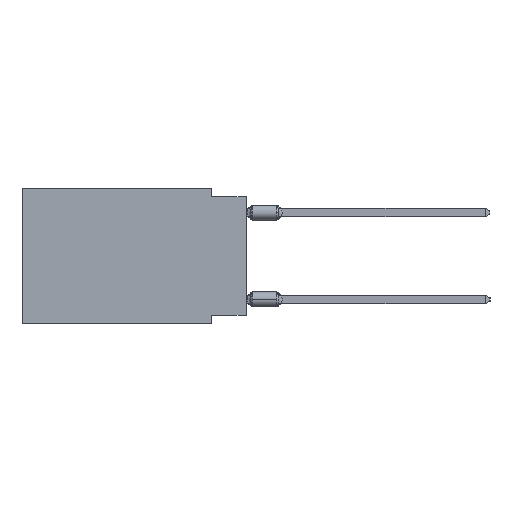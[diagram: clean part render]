
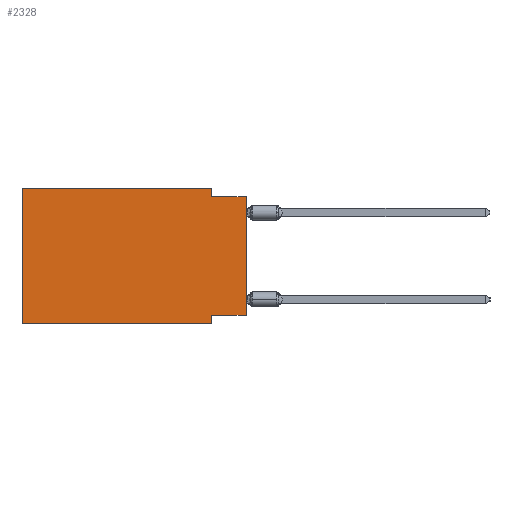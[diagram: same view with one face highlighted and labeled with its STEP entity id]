
A CAD part, left-side view. The second image highlights one B-rep face of the part: STEP entity #2328.
In plain terms, the highlighted planar face has unit normal (-1, 0, 0).
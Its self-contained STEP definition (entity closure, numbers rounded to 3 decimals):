
#2328 = ADVANCED_FACE ( 'NONE', ( #40410 ), #28018, .F. ) ;
#2558 = VECTOR ( 'NONE', #44856, 1000. ) ;
#3671 = CARTESIAN_POINT ( 'NONE',  ( 0., 0., 0. ) ) ;
#4469 = VECTOR ( 'NONE', #50687, 1000. ) ;
#4748 = VECTOR ( 'NONE', #26345, 1000. ) ;
#4907 = ORIENTED_EDGE ( 'NONE', *, *, #16165, .F. ) ;
#4925 = EDGE_CURVE ( 'NONE', #30814, #30671, #46472, .T. ) ;
#4970 = CARTESIAN_POINT ( 'NONE',  ( 0., 0., -0.635 ) ) ;
#5239 = VERTEX_POINT ( 'NONE', #12383 ) ;
#5665 = CARTESIAN_POINT ( 'NONE',  ( 0., 2.54, 0. ) ) ;
#8588 = DIRECTION ( 'NONE',  ( 0., -1., 0. ) ) ;
#9917 = VERTEX_POINT ( 'NONE', #5665 ) ;
#10770 = CARTESIAN_POINT ( 'NONE',  ( 0., 16.383, 0. ) ) ;
#11943 = VECTOR ( 'NONE', #44067, 1000. ) ;
#12214 = VERTEX_POINT ( 'NONE', #50685 ) ;
#12383 = CARTESIAN_POINT ( 'NONE',  ( 0., 0., -9.271 ) ) ;
#12492 = ORIENTED_EDGE ( 'NONE', *, *, #39696, .F. ) ;
#13173 = DIRECTION ( 'NONE',  ( 0., 0., -1. ) ) ;
#13959 = CARTESIAN_POINT ( 'NONE',  ( 0., 2.54, 0. ) ) ;
#14787 = CARTESIAN_POINT ( 'NONE',  ( 0., 0., -9.271 ) ) ;
#14812 = ORIENTED_EDGE ( 'NONE', *, *, #31121, .F. ) ;
#16165 = EDGE_CURVE ( 'NONE', #32740, #9917, #23938, .T. ) ;
#16722 = DIRECTION ( 'NONE',  ( 0., -1., 0. ) ) ;
#16912 = CARTESIAN_POINT ( 'NONE',  ( 0., 2.54, -9.906 ) ) ;
#17437 = CARTESIAN_POINT ( 'NONE',  ( 0., 2.54, -9.271 ) ) ;
#18923 = ORIENTED_EDGE ( 'NONE', *, *, #31008, .F. ) ;
#20093 = CARTESIAN_POINT ( 'NONE',  ( 0., 16.383, 0. ) ) ;
#20736 = CARTESIAN_POINT ( 'NONE',  ( 0., 16.383, 0. ) ) ;
#22912 = LINE ( 'NONE', #50898, #4748 ) ;
#23659 = EDGE_CURVE ( 'NONE', #5239, #39561, #35359, .T. ) ;
#23938 = LINE ( 'NONE', #20736, #32534 ) ;
#24519 = CARTESIAN_POINT ( 'NONE',  ( 0., 16.383, 0. ) ) ;
#24653 = LINE ( 'NONE', #41024, #50578 ) ;
#24776 = LINE ( 'NONE', #24519, #2558 ) ;
#26345 = DIRECTION ( 'NONE',  ( 0., -1., 0. ) ) ;
#26402 = DIRECTION ( 'NONE',  ( 0., 1., 0. ) ) ;
#28018 = PLANE ( 'NONE',  #42121 ) ;
#30471 = EDGE_LOOP ( 'NONE', ( #40165, #12492, #32996, #4907, #14812, #39745, #48028, #18923 ) ) ;
#30671 = VERTEX_POINT ( 'NONE', #16912 ) ;
#30814 = VERTEX_POINT ( 'NONE', #17437 ) ;
#31008 = EDGE_CURVE ( 'NONE', #5239, #30814, #46751, .T. ) ;
#31121 = EDGE_CURVE ( 'NONE', #41843, #32740, #24776, .T. ) ;
#32534 = VECTOR ( 'NONE', #8588, 1000. ) ;
#32740 = VERTEX_POINT ( 'NONE', #10770 ) ;
#32996 = ORIENTED_EDGE ( 'NONE', *, *, #44003, .F. ) ;
#35359 = LINE ( 'NONE', #3671, #11943 ) ;
#36618 = EDGE_CURVE ( 'NONE', #41843, #30671, #24653, .T. ) ;
#36717 = DIRECTION ( 'NONE',  ( 1., 0., 0. ) ) ;
#39561 = VERTEX_POINT ( 'NONE', #4970 ) ;
#39696 = EDGE_CURVE ( 'NONE', #12214, #39561, #22912, .T. ) ;
#39745 = ORIENTED_EDGE ( 'NONE', *, *, #36618, .T. ) ;
#40165 = ORIENTED_EDGE ( 'NONE', *, *, #23659, .T. ) ;
#40410 = FACE_OUTER_BOUND ( 'NONE', #30471, .T. ) ;
#41024 = CARTESIAN_POINT ( 'NONE',  ( 0., 16.383, -9.906 ) ) ;
#41145 = VECTOR ( 'NONE', #13173, 1000. ) ;
#41843 = VERTEX_POINT ( 'NONE', #52141 ) ;
#42121 = AXIS2_PLACEMENT_3D ( 'NONE', #20093, #36717, #43872 ) ;
#42215 = VECTOR ( 'NONE', #26402, 1000. ) ;
#42528 = CARTESIAN_POINT ( 'NONE',  ( 0., 2.54, -9.906 ) ) ;
#43872 = DIRECTION ( 'NONE',  ( 0., 0., -1. ) ) ;
#44003 = EDGE_CURVE ( 'NONE', #9917, #12214, #50143, .T. ) ;
#44067 = DIRECTION ( 'NONE',  ( 0., 0., 1. ) ) ;
#44856 = DIRECTION ( 'NONE',  ( 0., 0., 1. ) ) ;
#46472 = LINE ( 'NONE', #42528, #4469 ) ;
#46751 = LINE ( 'NONE', #14787, #42215 ) ;
#48028 = ORIENTED_EDGE ( 'NONE', *, *, #4925, .F. ) ;
#50143 = LINE ( 'NONE', #13959, #41145 ) ;
#50578 = VECTOR ( 'NONE', #16722, 1000. ) ;
#50685 = CARTESIAN_POINT ( 'NONE',  ( 0., 2.54, -0.635 ) ) ;
#50687 = DIRECTION ( 'NONE',  ( 0., 0., -1. ) ) ;
#50898 = CARTESIAN_POINT ( 'NONE',  ( 0., 0., -0.635 ) ) ;
#52141 = CARTESIAN_POINT ( 'NONE',  ( 0., 16.383, -9.906 ) ) ;
